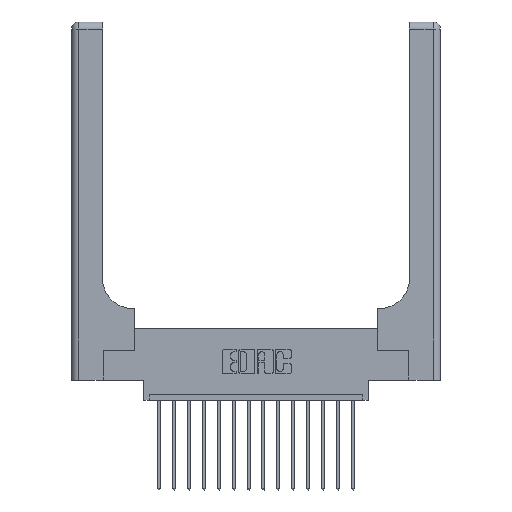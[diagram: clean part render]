
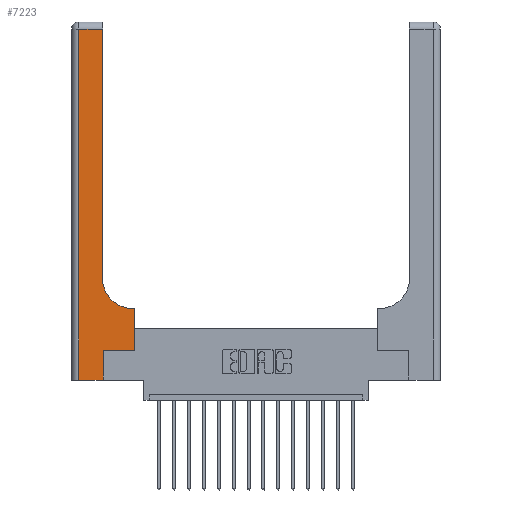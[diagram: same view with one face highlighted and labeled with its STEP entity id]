
A CAD part, top view. The second image highlights one B-rep face of the part: STEP entity #7223.
In plain terms, the highlighted planar face has unit normal (0, 0, 1).
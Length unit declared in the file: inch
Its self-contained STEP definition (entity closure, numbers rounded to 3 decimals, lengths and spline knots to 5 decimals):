
#49 = EDGE_LOOP ( 'NONE', ( #15155, #13764, #3460, #5606, #11744, #8096, #3761, #17497, #3693 ) ) ;
#522 = CARTESIAN_POINT ( 'NONE',  ( 0.265, 0.25, 0.37 ) ) ;
#710 = LINE ( 'NONE', #10096, #1144 ) ;
#782 = FACE_OUTER_BOUND ( 'NONE', #49, .T. ) ;
#1144 = VECTOR ( 'NONE', #12236, 39.37008 ) ;
#1209 = CARTESIAN_POINT ( 'NONE',  ( 0.26, 2.94, 0.37 ) ) ;
#1538 = VERTEX_POINT ( 'NONE', #6821 ) ;
#2298 = CIRCLE ( 'NONE', #16837, 0.25 ) ;
#2490 = CARTESIAN_POINT ( 'NONE',  ( 0.26, 0.85, 0.37 ) ) ;
#3097 = DIRECTION ( 'NONE',  ( -1., 0., 0. ) ) ;
#3216 = CARTESIAN_POINT ( 'NONE',  ( 0., 0., 0.37 ) ) ;
#3232 = VERTEX_POINT ( 'NONE', #10951 ) ;
#3285 = CARTESIAN_POINT ( 'NONE',  ( 0.265, 0., 0.37 ) ) ;
#3460 = ORIENTED_EDGE ( 'NONE', *, *, #15017, .T. ) ;
#3693 = ORIENTED_EDGE ( 'NONE', *, *, #12976, .T. ) ;
#3761 = ORIENTED_EDGE ( 'NONE', *, *, #11232, .T. ) ;
#4012 = DIRECTION ( 'NONE',  ( 1., 0., 0. ) ) ;
#4129 = VERTEX_POINT ( 'NONE', #3285 ) ;
#4352 = VERTEX_POINT ( 'NONE', #1209 ) ;
#4716 = CARTESIAN_POINT ( 'NONE',  ( 0.26, 0.6, 0.37 ) ) ;
#4986 = VERTEX_POINT ( 'NONE', #17396 ) ;
#5384 = CARTESIAN_POINT ( 'NONE',  ( 0.51, 0.85, 0.37 ) ) ;
#5533 = CARTESIAN_POINT ( 'NONE',  ( 0.06, 3., 0.37 ) ) ;
#5606 = ORIENTED_EDGE ( 'NONE', *, *, #8112, .T. ) ;
#5907 = CARTESIAN_POINT ( 'NONE',  ( 0.528, 0.25, 0.37 ) ) ;
#6086 = VECTOR ( 'NONE', #17082, 39.37008 ) ;
#6336 = VERTEX_POINT ( 'NONE', #6928 ) ;
#6468 = EDGE_CURVE ( 'NONE', #4986, #13151, #16932, .T. ) ;
#6507 = DIRECTION ( 'NONE',  ( 0., 0., -1. ) ) ;
#6821 = CARTESIAN_POINT ( 'NONE',  ( 0.528, 0.6, 0.37 ) ) ;
#6928 = CARTESIAN_POINT ( 'NONE',  ( 0.51, 0.6, 0.37 ) ) ;
#7223 = ADVANCED_FACE ( 'NONE', ( #782 ), #10658, .F. ) ;
#7782 = EDGE_CURVE ( 'NONE', #1538, #6336, #11538, .T. ) ;
#7937 = VERTEX_POINT ( 'NONE', #2490 ) ;
#8096 = ORIENTED_EDGE ( 'NONE', *, *, #6468, .T. ) ;
#8112 = EDGE_CURVE ( 'NONE', #3232, #4129, #11740, .T. ) ;
#8587 = VECTOR ( 'NONE', #12867, 39.37008 ) ;
#8592 = VERTEX_POINT ( 'NONE', #8760 ) ;
#8653 = EDGE_CURVE ( 'NONE', #7937, #4352, #710, .T. ) ;
#8687 = DIRECTION ( 'NONE',  ( 1., 0., 0. ) ) ;
#8760 = CARTESIAN_POINT ( 'NONE',  ( 0.06, 2.94, 0.37 ) ) ;
#8765 = DIRECTION ( 'NONE',  ( 1., 0., 0. ) ) ;
#9373 = DIRECTION ( 'NONE',  ( 0., 1., 0. ) ) ;
#9381 = VECTOR ( 'NONE', #8687, 39.37008 ) ;
#10096 = CARTESIAN_POINT ( 'NONE',  ( 0.26, 3., 0.37 ) ) ;
#10429 = LINE ( 'NONE', #5533, #12998 ) ;
#10658 = PLANE ( 'NONE',  #14250 ) ;
#10716 = CARTESIAN_POINT ( 'NONE',  ( 0., 3., 0.37 ) ) ;
#10951 = CARTESIAN_POINT ( 'NONE',  ( 0.06, 0., 0.37 ) ) ;
#10958 = LINE ( 'NONE', #5907, #8587 ) ;
#11232 = EDGE_CURVE ( 'NONE', #13151, #1538, #10958, .T. ) ;
#11538 = LINE ( 'NONE', #4716, #16466 ) ;
#11740 = LINE ( 'NONE', #3216, #9381 ) ;
#11744 = ORIENTED_EDGE ( 'NONE', *, *, #15602, .T. ) ;
#12126 = CARTESIAN_POINT ( 'NONE',  ( 0.265, 0., 0.37 ) ) ;
#12236 = DIRECTION ( 'NONE',  ( 0., 1., 0. ) ) ;
#12730 = CARTESIAN_POINT ( 'NONE',  ( 0.528, 0.25, 0.37 ) ) ;
#12867 = DIRECTION ( 'NONE',  ( 0., 1., 0. ) ) ;
#12976 = EDGE_CURVE ( 'NONE', #6336, #7937, #2298, .T. ) ;
#12998 = VECTOR ( 'NONE', #13777, 39.37008 ) ;
#13151 = VERTEX_POINT ( 'NONE', #12730 ) ;
#13471 = DIRECTION ( 'NONE',  ( -1., 0., 0. ) ) ;
#13506 = DIRECTION ( 'NONE',  ( 0., 0., -1. ) ) ;
#13764 = ORIENTED_EDGE ( 'NONE', *, *, #16042, .T. ) ;
#13777 = DIRECTION ( 'NONE',  ( 0., -1., 0. ) ) ;
#14250 = AXIS2_PLACEMENT_3D ( 'NONE', #10716, #6507, #13471 ) ;
#14262 = VECTOR ( 'NONE', #9373, 39.37008 ) ;
#15017 = EDGE_CURVE ( 'NONE', #8592, #3232, #10429, .T. ) ;
#15155 = ORIENTED_EDGE ( 'NONE', *, *, #8653, .T. ) ;
#15448 = VECTOR ( 'NONE', #8765, 39.37008 ) ;
#15602 = EDGE_CURVE ( 'NONE', #4129, #4986, #17457, .T. ) ;
#15927 = CARTESIAN_POINT ( 'NONE',  ( 0., 2.94, 0.37 ) ) ;
#16042 = EDGE_CURVE ( 'NONE', #4352, #8592, #17010, .T. ) ;
#16466 = VECTOR ( 'NONE', #3097, 39.37008 ) ;
#16837 = AXIS2_PLACEMENT_3D ( 'NONE', #5384, #13506, #4012 ) ;
#16932 = LINE ( 'NONE', #522, #15448 ) ;
#17010 = LINE ( 'NONE', #15927, #6086 ) ;
#17082 = DIRECTION ( 'NONE',  ( -1., 0., 0. ) ) ;
#17396 = CARTESIAN_POINT ( 'NONE',  ( 0.265, 0.25, 0.37 ) ) ;
#17457 = LINE ( 'NONE', #12126, #14262 ) ;
#17497 = ORIENTED_EDGE ( 'NONE', *, *, #7782, .T. ) ;
